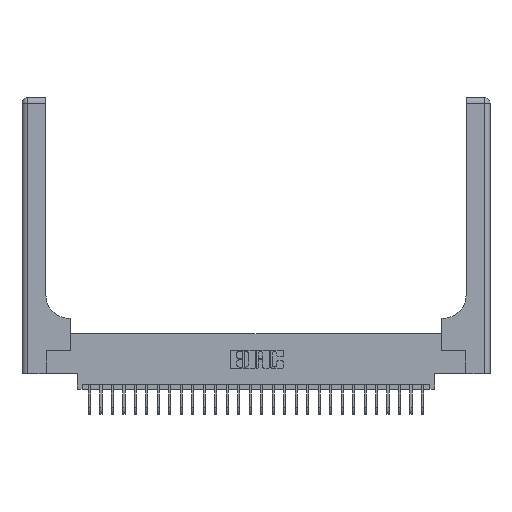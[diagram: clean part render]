
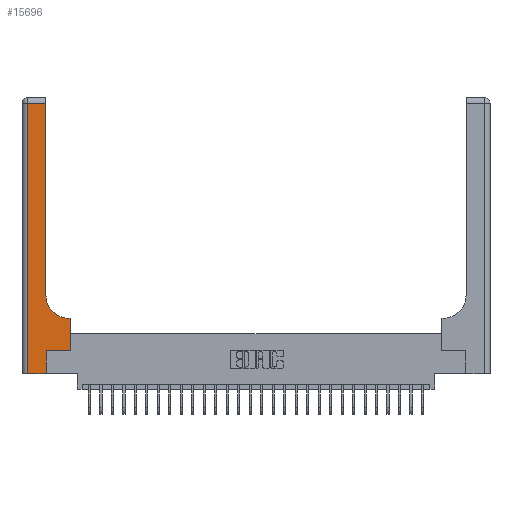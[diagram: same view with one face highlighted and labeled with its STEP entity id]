
A CAD part, top view. The second image highlights one B-rep face of the part: STEP entity #15696.
In plain terms, the highlighted planar face has unit normal (0, 0, 1).
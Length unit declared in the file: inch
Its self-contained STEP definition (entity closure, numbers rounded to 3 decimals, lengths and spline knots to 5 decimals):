
#492 = EDGE_LOOP ( 'NONE', ( #10921, #23357, #8713, #6486, #10051, #10257, #18484, #4297, #9925 ) ) ;
#610 = DIRECTION ( 'NONE',  ( 0., 0., -1. ) ) ;
#793 = CARTESIAN_POINT ( 'NONE',  ( 0.26, 3., 0.37 ) ) ;
#1058 = CARTESIAN_POINT ( 'NONE',  ( 0.265, 0., 0.37 ) ) ;
#1104 = VERTEX_POINT ( 'NONE', #13285 ) ;
#1345 = LINE ( 'NONE', #15711, #3969 ) ;
#1552 = LINE ( 'NONE', #11185, #16221 ) ;
#2064 = VERTEX_POINT ( 'NONE', #19408 ) ;
#2204 = DIRECTION ( 'NONE',  ( -1., 0., 0. ) ) ;
#2572 = CARTESIAN_POINT ( 'NONE',  ( 0.26, 0.85, 0.37 ) ) ;
#2639 = EDGE_CURVE ( 'NONE', #18964, #24238, #24590, .T. ) ;
#2718 = CARTESIAN_POINT ( 'NONE',  ( 0.51, 0.85, 0.37 ) ) ;
#3422 = CARTESIAN_POINT ( 'NONE',  ( 0.528, 0.25, 0.37 ) ) ;
#3969 = VECTOR ( 'NONE', #25466, 39.37008 ) ;
#4297 = ORIENTED_EDGE ( 'NONE', *, *, #11013, .T. ) ;
#4485 = DIRECTION ( 'NONE',  ( 0., 1., 0. ) ) ;
#4516 = EDGE_CURVE ( 'NONE', #12968, #5879, #1345, .T. ) ;
#5025 = VECTOR ( 'NONE', #14599, 39.37008 ) ;
#5360 = VERTEX_POINT ( 'NONE', #2572 ) ;
#5585 = DIRECTION ( 'NONE',  ( -1., 0., 0. ) ) ;
#5879 = VERTEX_POINT ( 'NONE', #21354 ) ;
#6205 = EDGE_CURVE ( 'NONE', #15847, #18964, #1552, .T. ) ;
#6469 = LINE ( 'NONE', #793, #15444 ) ;
#6486 = ORIENTED_EDGE ( 'NONE', *, *, #4516, .T. ) ;
#6489 = LINE ( 'NONE', #1058, #6617 ) ;
#6617 = VECTOR ( 'NONE', #18720, 39.37008 ) ;
#7079 = CARTESIAN_POINT ( 'NONE',  ( 0.528, 0.6, 0.37 ) ) ;
#7382 = AXIS2_PLACEMENT_3D ( 'NONE', #17310, #15324, #5585 ) ;
#7531 = CARTESIAN_POINT ( 'NONE',  ( 0.06, 0., 0.37 ) ) ;
#7739 = EDGE_CURVE ( 'NONE', #5879, #15847, #6489, .T. ) ;
#8713 = ORIENTED_EDGE ( 'NONE', *, *, #11994, .T. ) ;
#9291 = FACE_OUTER_BOUND ( 'NONE', #492, .T. ) ;
#9867 = EDGE_CURVE ( 'NONE', #2064, #5360, #16705, .T. ) ;
#9925 = ORIENTED_EDGE ( 'NONE', *, *, #9867, .T. ) ;
#10051 = ORIENTED_EDGE ( 'NONE', *, *, #7739, .T. ) ;
#10257 = ORIENTED_EDGE ( 'NONE', *, *, #6205, .T. ) ;
#10394 = LINE ( 'NONE', #14457, #20497 ) ;
#10517 = CARTESIAN_POINT ( 'NONE',  ( 0.528, 0.25, 0.37 ) ) ;
#10654 = VERTEX_POINT ( 'NONE', #12393 ) ;
#10921 = ORIENTED_EDGE ( 'NONE', *, *, #11591, .T. ) ;
#11013 = EDGE_CURVE ( 'NONE', #24238, #2064, #15282, .T. ) ;
#11185 = CARTESIAN_POINT ( 'NONE',  ( 0.265, 0.25, 0.37 ) ) ;
#11591 = EDGE_CURVE ( 'NONE', #5360, #1104, #6469, .T. ) ;
#11994 = EDGE_CURVE ( 'NONE', #10654, #12968, #10394, .T. ) ;
#12018 = LINE ( 'NONE', #20923, #5025 ) ;
#12359 = CARTESIAN_POINT ( 'NONE',  ( 0.26, 0.6, 0.37 ) ) ;
#12393 = CARTESIAN_POINT ( 'NONE',  ( 0.06, 2.94, 0.37 ) ) ;
#12968 = VERTEX_POINT ( 'NONE', #7531 ) ;
#13285 = CARTESIAN_POINT ( 'NONE',  ( 0.26, 2.94, 0.37 ) ) ;
#13675 = DIRECTION ( 'NONE',  ( 1., 0., 0. ) ) ;
#14457 = CARTESIAN_POINT ( 'NONE',  ( 0.06, 3., 0.37 ) ) ;
#14502 = EDGE_CURVE ( 'NONE', #1104, #10654, #12018, .T. ) ;
#14599 = DIRECTION ( 'NONE',  ( -1., 0., 0. ) ) ;
#15282 = LINE ( 'NONE', #12359, #21307 ) ;
#15324 = DIRECTION ( 'NONE',  ( 0., 0., -1. ) ) ;
#15444 = VECTOR ( 'NONE', #4485, 39.37008 ) ;
#15696 = ADVANCED_FACE ( 'NONE', ( #9291 ), #23766, .F. ) ;
#15711 = CARTESIAN_POINT ( 'NONE',  ( 0., 0., 0.37 ) ) ;
#15847 = VERTEX_POINT ( 'NONE', #15855 ) ;
#15855 = CARTESIAN_POINT ( 'NONE',  ( 0.265, 0.25, 0.37 ) ) ;
#16221 = VECTOR ( 'NONE', #13675, 39.37008 ) ;
#16705 = CIRCLE ( 'NONE', #23438, 0.25 ) ;
#17310 = CARTESIAN_POINT ( 'NONE',  ( 0., 3., 0.37 ) ) ;
#18484 = ORIENTED_EDGE ( 'NONE', *, *, #2639, .T. ) ;
#18534 = DIRECTION ( 'NONE',  ( 0., 1., 0. ) ) ;
#18720 = DIRECTION ( 'NONE',  ( 0., 1., 0. ) ) ;
#18964 = VERTEX_POINT ( 'NONE', #3422 ) ;
#19082 = VECTOR ( 'NONE', #18534, 39.37008 ) ;
#19408 = CARTESIAN_POINT ( 'NONE',  ( 0.51, 0.6, 0.37 ) ) ;
#20497 = VECTOR ( 'NONE', #22765, 39.37008 ) ;
#20774 = DIRECTION ( 'NONE',  ( 1., 0., 0. ) ) ;
#20923 = CARTESIAN_POINT ( 'NONE',  ( 0., 2.94, 0.37 ) ) ;
#21307 = VECTOR ( 'NONE', #2204, 39.37008 ) ;
#21354 = CARTESIAN_POINT ( 'NONE',  ( 0.265, 0., 0.37 ) ) ;
#22765 = DIRECTION ( 'NONE',  ( 0., -1., 0. ) ) ;
#23357 = ORIENTED_EDGE ( 'NONE', *, *, #14502, .T. ) ;
#23438 = AXIS2_PLACEMENT_3D ( 'NONE', #2718, #610, #20774 ) ;
#23766 = PLANE ( 'NONE',  #7382 ) ;
#24238 = VERTEX_POINT ( 'NONE', #7079 ) ;
#24590 = LINE ( 'NONE', #10517, #19082 ) ;
#25466 = DIRECTION ( 'NONE',  ( 1., 0., 0. ) ) ;
